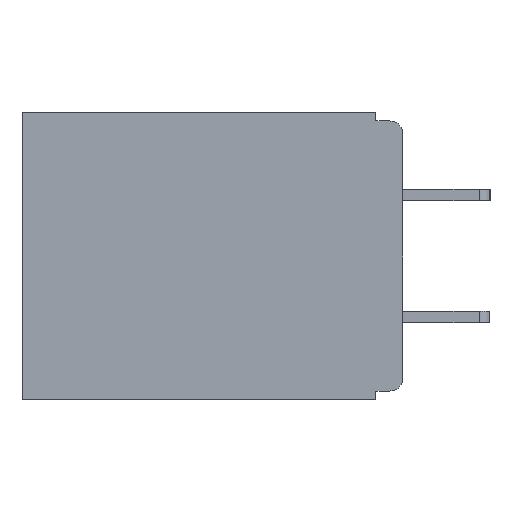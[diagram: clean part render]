
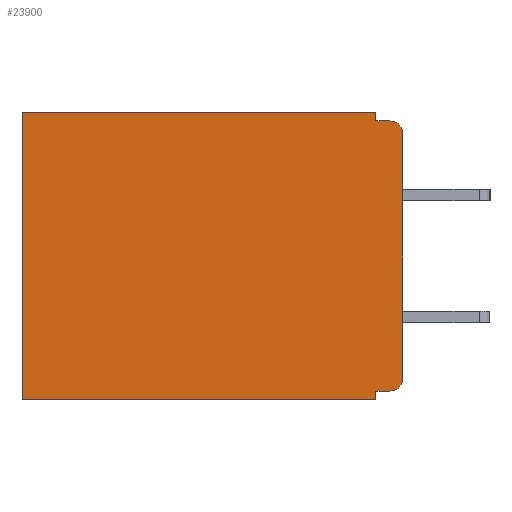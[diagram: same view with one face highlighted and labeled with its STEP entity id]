
A CAD part, left-side view. The second image highlights one B-rep face of the part: STEP entity #23900.
In plain terms, the highlighted planar face has unit normal (-1, 0, 0).
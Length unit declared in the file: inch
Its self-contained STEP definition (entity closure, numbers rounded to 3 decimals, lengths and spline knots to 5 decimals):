
#1202 = VECTOR ( 'NONE', #5774, 39.37008 ) ;
#1274 = CARTESIAN_POINT ( 'NONE',  ( 0.3, 0., -0.01 ) ) ;
#1309 = AXIS2_PLACEMENT_3D ( 'NONE', #12129, #3598, #18866 ) ;
#1443 = EDGE_CURVE ( 'NONE', #19062, #18193, #17457, .T. ) ;
#2168 = DIRECTION ( 'NONE',  ( -1., 0., 0. ) ) ;
#2336 = LINE ( 'NONE', #26747, #15865 ) ;
#3598 = DIRECTION ( 'NONE',  ( 1., 0., 0. ) ) ;
#3920 = VERTEX_POINT ( 'NONE', #25019 ) ;
#4004 = VERTEX_POINT ( 'NONE', #24988 ) ;
#4016 = VECTOR ( 'NONE', #14190, 39.37008 ) ;
#4849 = VERTEX_POINT ( 'NONE', #22425 ) ;
#5258 = CARTESIAN_POINT ( 'NONE',  ( 0.3, 0., -0.305 ) ) ;
#5409 = DIRECTION ( 'NONE',  ( 0., 0., -1. ) ) ;
#5502 = DIRECTION ( 'NONE',  ( 0., 1., 0. ) ) ;
#5774 = DIRECTION ( 'NONE',  ( 0., 0., -1. ) ) ;
#5831 = VECTOR ( 'NONE', #16984, 39.37008 ) ;
#6137 = AXIS2_PLACEMENT_3D ( 'NONE', #21227, #8099, #23407 ) ;
#6605 = CIRCLE ( 'NONE', #18303, 0.015 ) ;
#6868 = LINE ( 'NONE', #16603, #1202 ) ;
#7313 = CARTESIAN_POINT ( 'NONE',  ( 0.3, 0., -0.33 ) ) ;
#7330 = EDGE_CURVE ( 'NONE', #21442, #24433, #12847, .T. ) ;
#7374 = EDGE_CURVE ( 'NONE', #3920, #13802, #12149, .T. ) ;
#7508 = CARTESIAN_POINT ( 'NONE',  ( 0.3, 0.437, 0. ) ) ;
#8099 = DIRECTION ( 'NONE',  ( -1., 0., 0. ) ) ;
#10674 = EDGE_CURVE ( 'NONE', #4004, #24433, #18933, .T. ) ;
#10883 = CARTESIAN_POINT ( 'NONE',  ( 0.3, 0., -0.32 ) ) ;
#10997 = ORIENTED_EDGE ( 'NONE', *, *, #1443, .F. ) ;
#11835 = EDGE_CURVE ( 'NONE', #18193, #24377, #23544, .T. ) ;
#12046 = VECTOR ( 'NONE', #13119, 39.37008 ) ;
#12092 = ORIENTED_EDGE ( 'NONE', *, *, #14010, .T. ) ;
#12129 = CARTESIAN_POINT ( 'NONE',  ( 0.3, 0., -0.33 ) ) ;
#12149 = LINE ( 'NONE', #22812, #23793 ) ;
#12235 = EDGE_LOOP ( 'NONE', ( #23396, #12092, #13154, #21921, #17558, #23087, #18607, #10997, #26948, #27118 ) ) ;
#12564 = VERTEX_POINT ( 'NONE', #24955 ) ;
#12566 = CARTESIAN_POINT ( 'NONE',  ( 0.3, 0.031, -0.33 ) ) ;
#12847 = LINE ( 'NONE', #18496, #24434 ) ;
#13119 = DIRECTION ( 'NONE',  ( 0., 1., 0. ) ) ;
#13154 = ORIENTED_EDGE ( 'NONE', *, *, #13300, .F. ) ;
#13300 = EDGE_CURVE ( 'NONE', #12564, #4849, #14831, .T. ) ;
#13600 = CARTESIAN_POINT ( 'NONE',  ( 0.3, 0.031, -0.33 ) ) ;
#13802 = VERTEX_POINT ( 'NONE', #7508 ) ;
#13809 = DIRECTION ( 'NONE',  ( 0., 0., -1. ) ) ;
#14010 = EDGE_CURVE ( 'NONE', #21442, #4849, #6605, .T. ) ;
#14190 = DIRECTION ( 'NONE',  ( 0., -1., 0. ) ) ;
#14831 = LINE ( 'NONE', #1274, #4016 ) ;
#15101 = CARTESIAN_POINT ( 'NONE',  ( 0.3, 0.015, -0.025 ) ) ;
#15132 = EDGE_CURVE ( 'NONE', #13802, #24377, #6868, .T. ) ;
#15851 = CARTESIAN_POINT ( 'NONE',  ( 0.3, 0.437, -0.33 ) ) ;
#15865 = VECTOR ( 'NONE', #13809, 39.37008 ) ;
#16578 = PLANE ( 'NONE',  #1309 ) ;
#16603 = CARTESIAN_POINT ( 'NONE',  ( 0.3, 0.437, -0.33 ) ) ;
#16984 = DIRECTION ( 'NONE',  ( 0., 0., -1. ) ) ;
#17389 = DIRECTION ( 'NONE',  ( 0., 0., -1. ) ) ;
#17457 = LINE ( 'NONE', #12566, #5831 ) ;
#17558 = ORIENTED_EDGE ( 'NONE', *, *, #7374, .T. ) ;
#17809 = VECTOR ( 'NONE', #20454, 39.37008 ) ;
#18193 = VERTEX_POINT ( 'NONE', #13600 ) ;
#18303 = AXIS2_PLACEMENT_3D ( 'NONE', #15101, #2168, #17389 ) ;
#18496 = CARTESIAN_POINT ( 'NONE',  ( 0.3, 0., -0.33 ) ) ;
#18607 = ORIENTED_EDGE ( 'NONE', *, *, #11835, .F. ) ;
#18866 = DIRECTION ( 'NONE',  ( 0., 0., -1. ) ) ;
#18933 = CIRCLE ( 'NONE', #6137, 0.015 ) ;
#19062 = VERTEX_POINT ( 'NONE', #27318 ) ;
#20454 = DIRECTION ( 'NONE',  ( 0., 1., 0. ) ) ;
#21227 = CARTESIAN_POINT ( 'NONE',  ( 0.3, 0.015, -0.305 ) ) ;
#21442 = VERTEX_POINT ( 'NONE', #27584 ) ;
#21921 = ORIENTED_EDGE ( 'NONE', *, *, #23074, .F. ) ;
#22425 = CARTESIAN_POINT ( 'NONE',  ( 0.3, 0.015, -0.01 ) ) ;
#22812 = CARTESIAN_POINT ( 'NONE',  ( 0.3, 0., 0. ) ) ;
#23074 = EDGE_CURVE ( 'NONE', #3920, #12564, #2336, .T. ) ;
#23087 = ORIENTED_EDGE ( 'NONE', *, *, #15132, .T. ) ;
#23396 = ORIENTED_EDGE ( 'NONE', *, *, #7330, .F. ) ;
#23407 = DIRECTION ( 'NONE',  ( 0., 0., -1. ) ) ;
#23544 = LINE ( 'NONE', #7313, #17809 ) ;
#23793 = VECTOR ( 'NONE', #5502, 39.37008 ) ;
#23900 = ADVANCED_FACE ( 'NONE', ( #25646 ), #16578, .F. ) ;
#24377 = VERTEX_POINT ( 'NONE', #15851 ) ;
#24433 = VERTEX_POINT ( 'NONE', #5258 ) ;
#24434 = VECTOR ( 'NONE', #5409, 39.37008 ) ;
#24955 = CARTESIAN_POINT ( 'NONE',  ( 0.3, 0.031, -0.01 ) ) ;
#24988 = CARTESIAN_POINT ( 'NONE',  ( 0.3, 0.015, -0.32 ) ) ;
#25019 = CARTESIAN_POINT ( 'NONE',  ( 0.3, 0.031, 0. ) ) ;
#25646 = FACE_OUTER_BOUND ( 'NONE', #12235, .T. ) ;
#26747 = CARTESIAN_POINT ( 'NONE',  ( 0.3, 0.031, 0. ) ) ;
#26948 = ORIENTED_EDGE ( 'NONE', *, *, #27895, .F. ) ;
#27118 = ORIENTED_EDGE ( 'NONE', *, *, #10674, .T. ) ;
#27318 = CARTESIAN_POINT ( 'NONE',  ( 0.3, 0.031, -0.32 ) ) ;
#27584 = CARTESIAN_POINT ( 'NONE',  ( 0.3, 0., -0.025 ) ) ;
#27895 = EDGE_CURVE ( 'NONE', #4004, #19062, #27908, .T. ) ;
#27908 = LINE ( 'NONE', #10883, #12046 ) ;
